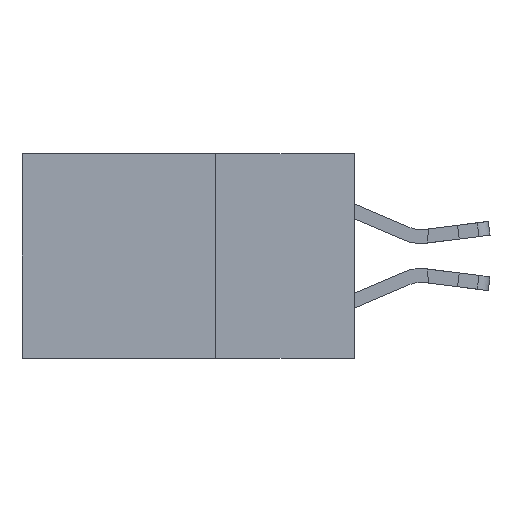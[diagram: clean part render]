
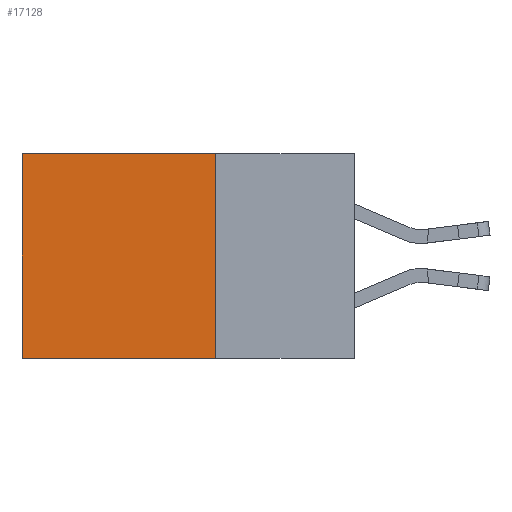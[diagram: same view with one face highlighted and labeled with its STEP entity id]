
A CAD part, left-side view. The second image highlights one B-rep face of the part: STEP entity #17128.
In plain terms, the highlighted planar face has unit normal (-1, 0, 0).
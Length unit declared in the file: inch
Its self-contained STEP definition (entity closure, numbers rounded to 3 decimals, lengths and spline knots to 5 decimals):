
#323 = VECTOR ( 'NONE', #2188, 39.37008 ) ;
#1786 = VERTEX_POINT ( 'NONE', #4553 ) ;
#2188 = DIRECTION ( 'NONE',  ( 0., 1., 0. ) ) ;
#2253 = CARTESIAN_POINT ( 'NONE',  ( 0.298, 0.25, 0. ) ) ;
#2692 = EDGE_CURVE ( 'NONE', #17318, #1786, #15035, .T. ) ;
#3136 = DIRECTION ( 'NONE',  ( 1., 0., 0. ) ) ;
#3609 = CARTESIAN_POINT ( 'NONE',  ( 0.298, 0.25, 0. ) ) ;
#3814 = LINE ( 'NONE', #2253, #323 ) ;
#4487 = CARTESIAN_POINT ( 'NONE',  ( 0.298, 0.25, -0.37 ) ) ;
#4553 = CARTESIAN_POINT ( 'NONE',  ( 0.298, 0.25, -0.37 ) ) ;
#4743 = CARTESIAN_POINT ( 'NONE',  ( 0.298, 0.6, 0. ) ) ;
#5546 = VERTEX_POINT ( 'NONE', #12754 ) ;
#5708 = EDGE_CURVE ( 'NONE', #17318, #5546, #3814, .T. ) ;
#6213 = EDGE_CURVE ( 'NONE', #5546, #14711, #14432, .T. ) ;
#6363 = VECTOR ( 'NONE', #15323, 39.37008 ) ;
#7723 = DIRECTION ( 'NONE',  ( 0., 0., -1. ) ) ;
#8071 = EDGE_CURVE ( 'NONE', #1786, #14711, #16831, .T. ) ;
#8842 = ORIENTED_EDGE ( 'NONE', *, *, #2692, .F. ) ;
#8917 = VECTOR ( 'NONE', #13599, 39.37008 ) ;
#9169 = CARTESIAN_POINT ( 'NONE',  ( 0.298, 0.25, 0. ) ) ;
#10164 = CARTESIAN_POINT ( 'NONE',  ( 0.298, 0.6, -0.37 ) ) ;
#11048 = VECTOR ( 'NONE', #7723, 39.37008 ) ;
#12244 = PLANE ( 'NONE',  #17714 ) ;
#12754 = CARTESIAN_POINT ( 'NONE',  ( 0.298, 0.6, 0. ) ) ;
#13599 = DIRECTION ( 'NONE',  ( 0., 1., 0. ) ) ;
#13728 = ORIENTED_EDGE ( 'NONE', *, *, #8071, .F. ) ;
#13753 = DIRECTION ( 'NONE',  ( 0., 0., -1. ) ) ;
#14024 = ORIENTED_EDGE ( 'NONE', *, *, #6213, .T. ) ;
#14432 = LINE ( 'NONE', #4743, #6363 ) ;
#14711 = VERTEX_POINT ( 'NONE', #10164 ) ;
#15035 = LINE ( 'NONE', #18892, #11048 ) ;
#15323 = DIRECTION ( 'NONE',  ( 0., 0., -1. ) ) ;
#16427 = ORIENTED_EDGE ( 'NONE', *, *, #5708, .T. ) ;
#16831 = LINE ( 'NONE', #4487, #8917 ) ;
#17128 = ADVANCED_FACE ( 'NONE', ( #17457 ), #12244, .F. ) ;
#17318 = VERTEX_POINT ( 'NONE', #3609 ) ;
#17375 = EDGE_LOOP ( 'NONE', ( #14024, #13728, #8842, #16427 ) ) ;
#17457 = FACE_OUTER_BOUND ( 'NONE', #17375, .T. ) ;
#17714 = AXIS2_PLACEMENT_3D ( 'NONE', #9169, #3136, #13753 ) ;
#18892 = CARTESIAN_POINT ( 'NONE',  ( 0.298, 0.25, 0. ) ) ;
